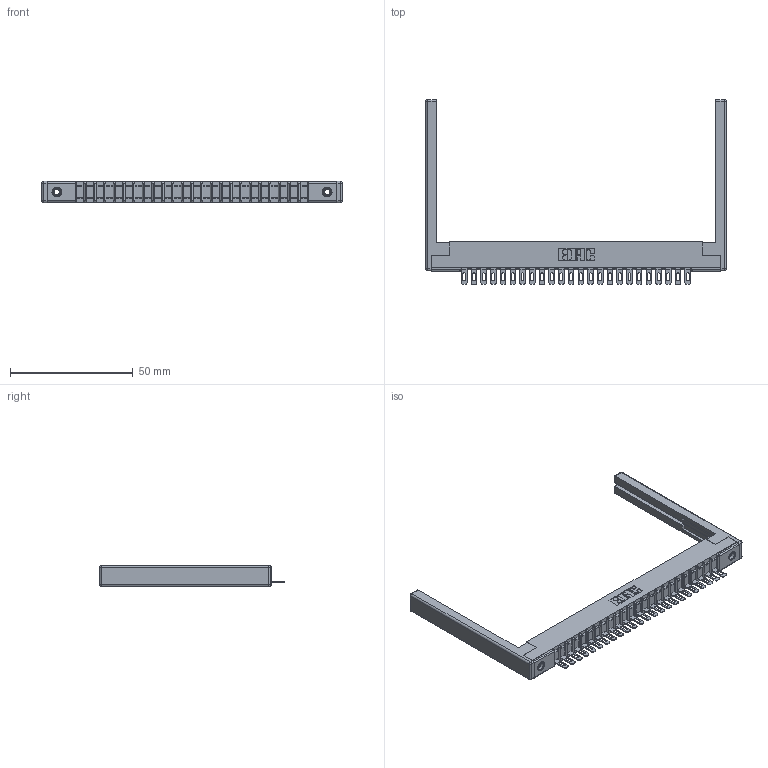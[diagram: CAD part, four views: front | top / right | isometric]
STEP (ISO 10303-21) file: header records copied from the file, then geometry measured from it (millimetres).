
FILE_DESCRIPTION (( 'STEP AP203' ), '1' );
FILE_NAME ('307-024-501-168.STEP', '2019-09-05T00:53:08', ( '' ), ( '' ), 'SwSTEP 2.0', 'SolidWorks 2016', '' );
FILE_SCHEMA (( 'CONFIG_CONTROL_DESIGN' ));
Length unit declared in the file: inch
Products named in the file (5): 307-220-068; 307 Part_.156 Dia Mounting Holes; 345-250-001_345-250-001-102; 307-290-002_501; 307-024-501-168
Assembly tree (29 placements, depth 2):
  307-024-501-168
    307 Part_.156 Dia Mounting Holes
    307-290-002_501  x24
    307-220-068  x2
    345-250-001_345-250-001-102  x2
Bounding box: 122.53 x 75.39 x 8.71 mm (x, y, z)
Volume: 12669.9 mm3; surface area: 19046.1 mm2
Topology: 29 solids, 29 shells, 2121 faces, 6425 edges, 4194 vertices
Faces by surface type: plane 1214, cylinder 833, sphere 58, cone 12, torus 4
Entity records: 26347 total; most frequent: CARTESIAN_POINT 4405, ORIENTED_EDGE 4384, DIRECTION 4310, EDGE_CURVE 2192, LINE 1664, VECTOR 1664, VERTEX_POINT 1418, AXIS2_PLACEMENT_3D 1323
